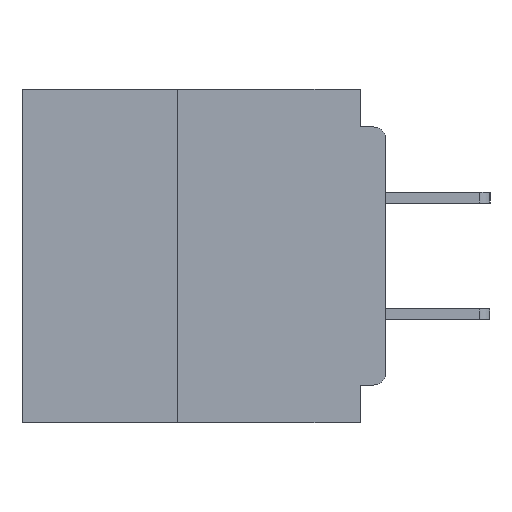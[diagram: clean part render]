
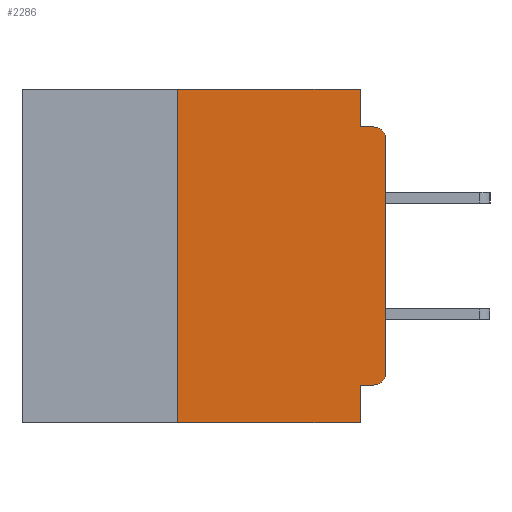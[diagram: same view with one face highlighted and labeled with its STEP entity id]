
A CAD part, left-side view. The second image highlights one B-rep face of the part: STEP entity #2286.
In plain terms, the highlighted planar face has unit normal (-1, 0, 0).
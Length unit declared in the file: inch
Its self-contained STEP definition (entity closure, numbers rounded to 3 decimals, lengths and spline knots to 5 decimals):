
#35 = CARTESIAN_POINT ( 'NONE',  ( 0., 0., -0.06 ) ) ;
#909 = VERTEX_POINT ( 'NONE', #36037 ) ;
#1753 = EDGE_CURVE ( 'NONE', #909, #31856, #40604, .T. ) ;
#2286 = ADVANCED_FACE ( 'NONE', ( #18981 ), #28272, .F. ) ;
#2800 = EDGE_CURVE ( 'NONE', #28062, #21531, #34203, .T. ) ;
#5672 = CARTESIAN_POINT ( 'NONE',  ( 0., 0.031, -0.4 ) ) ;
#5856 = DIRECTION ( 'NONE',  ( 0., 0., 1. ) ) ;
#5968 = CARTESIAN_POINT ( 'NONE',  ( 0., 0.25, -0.4 ) ) ;
#6632 = DIRECTION ( 'NONE',  ( -1., 0., 0. ) ) ;
#7144 = VERTEX_POINT ( 'NONE', #45603 ) ;
#7959 = VECTOR ( 'NONE', #47064, 39.37008 ) ;
#8208 = VERTEX_POINT ( 'NONE', #22354 ) ;
#8463 = CARTESIAN_POINT ( 'NONE',  ( 0., 0., -0.34 ) ) ;
#8759 = VECTOR ( 'NONE', #22665, 39.37008 ) ;
#9912 = LINE ( 'NONE', #39687, #38768 ) ;
#9921 = LINE ( 'NONE', #37515, #8759 ) ;
#10036 = LINE ( 'NONE', #31421, #48781 ) ;
#10285 = VECTOR ( 'NONE', #24651, 39.37008 ) ;
#11633 = ORIENTED_EDGE ( 'NONE', *, *, #41298, .T. ) ;
#12561 = CARTESIAN_POINT ( 'NONE',  ( 0., 0.031, -0.4 ) ) ;
#13236 = CARTESIAN_POINT ( 'NONE',  ( 0., 0.437, 0. ) ) ;
#13415 = DIRECTION ( 'NONE',  ( 0., 0., -1. ) ) ;
#13824 = EDGE_CURVE ( 'NONE', #8208, #44032, #10036, .T. ) ;
#14426 = VERTEX_POINT ( 'NONE', #12561 ) ;
#15400 = ORIENTED_EDGE ( 'NONE', *, *, #13824, .F. ) ;
#16542 = VERTEX_POINT ( 'NONE', #23448 ) ;
#16565 = VECTOR ( 'NONE', #40764, 39.37008 ) ;
#16803 = AXIS2_PLACEMENT_3D ( 'NONE', #19759, #45874, #23557 ) ;
#18517 = EDGE_CURVE ( 'NONE', #45107, #14426, #37984, .T. ) ;
#18981 = FACE_OUTER_BOUND ( 'NONE', #30210, .T. ) ;
#19759 = CARTESIAN_POINT ( 'NONE',  ( 0., 0.015, -0.06 ) ) ;
#20035 = CARTESIAN_POINT ( 'NONE',  ( 0., 0.031, -0.355 ) ) ;
#20331 = EDGE_CURVE ( 'NONE', #909, #14426, #27918, .T. ) ;
#21531 = VERTEX_POINT ( 'NONE', #35 ) ;
#22354 = CARTESIAN_POINT ( 'NONE',  ( 0., 0.031, -0.045 ) ) ;
#22665 = DIRECTION ( 'NONE',  ( 0., 1., 0. ) ) ;
#23448 = CARTESIAN_POINT ( 'NONE',  ( 0., 0.015, -0.355 ) ) ;
#23557 = DIRECTION ( 'NONE',  ( 0., 0., -1. ) ) ;
#24651 = DIRECTION ( 'NONE',  ( 0., -1., 0. ) ) ;
#24951 = EDGE_CURVE ( 'NONE', #16542, #28062, #31600, .T. ) ;
#25431 = EDGE_CURVE ( 'NONE', #31856, #7144, #32738, .T. ) ;
#26493 = DIRECTION ( 'NONE',  ( 0., 0., -1. ) ) ;
#26653 = DIRECTION ( 'NONE',  ( 1., 0., 0. ) ) ;
#27598 = CARTESIAN_POINT ( 'NONE',  ( 0., 0.437, 0. ) ) ;
#27886 = ORIENTED_EDGE ( 'NONE', *, *, #36730, .F. ) ;
#27918 = LINE ( 'NONE', #34893, #46513 ) ;
#28062 = VERTEX_POINT ( 'NONE', #8463 ) ;
#28104 = ORIENTED_EDGE ( 'NONE', *, *, #20331, .T. ) ;
#28272 = PLANE ( 'NONE',  #40313 ) ;
#29300 = CARTESIAN_POINT ( 'NONE',  ( 0., 0.015, -0.34 ) ) ;
#29538 = ORIENTED_EDGE ( 'NONE', *, *, #2800, .T. ) ;
#30158 = AXIS2_PLACEMENT_3D ( 'NONE', #29300, #6632, #33042 ) ;
#30210 = EDGE_LOOP ( 'NONE', ( #29538, #11633, #15400, #27886, #46133, #40741, #28104, #45769, #37808, #35916 ) ) ;
#30737 = VECTOR ( 'NONE', #5856, 39.37008 ) ;
#31421 = CARTESIAN_POINT ( 'NONE',  ( 0., 0., -0.045 ) ) ;
#31600 = CIRCLE ( 'NONE', #30158, 0.015 ) ;
#31856 = VERTEX_POINT ( 'NONE', #45089 ) ;
#32516 = CIRCLE ( 'NONE', #16803, 0.015 ) ;
#32738 = LINE ( 'NONE', #13236, #10285 ) ;
#33042 = DIRECTION ( 'NONE',  ( 0., 0., -1. ) ) ;
#34203 = LINE ( 'NONE', #40825, #16565 ) ;
#34893 = CARTESIAN_POINT ( 'NONE',  ( 0., 0.437, -0.4 ) ) ;
#35916 = ORIENTED_EDGE ( 'NONE', *, *, #24951, .T. ) ;
#36037 = CARTESIAN_POINT ( 'NONE',  ( 0., 0.25, -0.4 ) ) ;
#36730 = EDGE_CURVE ( 'NONE', #7144, #8208, #9912, .T. ) ;
#37515 = CARTESIAN_POINT ( 'NONE',  ( 0., 0., -0.355 ) ) ;
#37808 = ORIENTED_EDGE ( 'NONE', *, *, #43318, .F. ) ;
#37984 = LINE ( 'NONE', #5672, #7959 ) ;
#38768 = VECTOR ( 'NONE', #13415, 39.37008 ) ;
#38903 = DIRECTION ( 'NONE',  ( 0., -1., 0. ) ) ;
#39687 = CARTESIAN_POINT ( 'NONE',  ( 0., 0.031, 0. ) ) ;
#40313 = AXIS2_PLACEMENT_3D ( 'NONE', #27598, #26653, #26493 ) ;
#40604 = LINE ( 'NONE', #5968, #30737 ) ;
#40741 = ORIENTED_EDGE ( 'NONE', *, *, #1753, .F. ) ;
#40764 = DIRECTION ( 'NONE',  ( 0., 0., 1. ) ) ;
#40825 = CARTESIAN_POINT ( 'NONE',  ( 0., 0., 0. ) ) ;
#41298 = EDGE_CURVE ( 'NONE', #21531, #44032, #32516, .T. ) ;
#41701 = CARTESIAN_POINT ( 'NONE',  ( 0., 0.015, -0.045 ) ) ;
#43318 = EDGE_CURVE ( 'NONE', #16542, #45107, #9921, .T. ) ;
#44032 = VERTEX_POINT ( 'NONE', #41701 ) ;
#45089 = CARTESIAN_POINT ( 'NONE',  ( 0., 0.25, 0. ) ) ;
#45107 = VERTEX_POINT ( 'NONE', #20035 ) ;
#45603 = CARTESIAN_POINT ( 'NONE',  ( 0., 0.031, 0. ) ) ;
#45769 = ORIENTED_EDGE ( 'NONE', *, *, #18517, .F. ) ;
#45874 = DIRECTION ( 'NONE',  ( -1., 0., 0. ) ) ;
#46080 = DIRECTION ( 'NONE',  ( 0., -1., 0. ) ) ;
#46133 = ORIENTED_EDGE ( 'NONE', *, *, #25431, .F. ) ;
#46513 = VECTOR ( 'NONE', #46080, 39.37008 ) ;
#47064 = DIRECTION ( 'NONE',  ( 0., 0., -1. ) ) ;
#48781 = VECTOR ( 'NONE', #38903, 39.37008 ) ;
